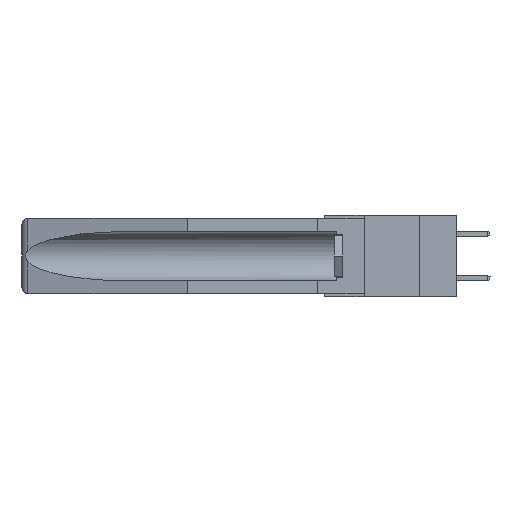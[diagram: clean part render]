
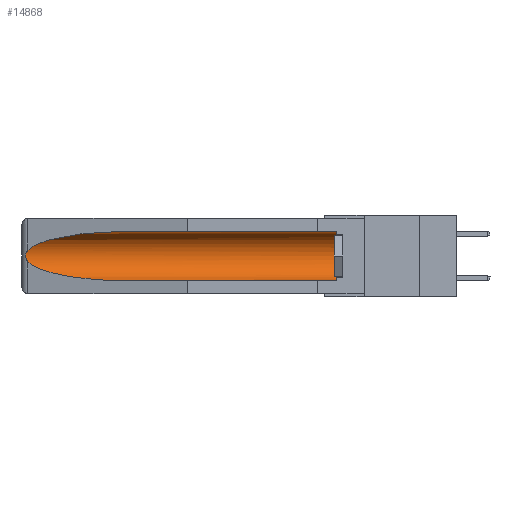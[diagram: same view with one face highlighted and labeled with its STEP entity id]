
A CAD part, left-side view. The second image highlights one B-rep face of the part: STEP entity #14868.
In plain terms, the highlighted cylindrical face has radius 2.857 mm (diameter 5.715 mm), a partial arc.
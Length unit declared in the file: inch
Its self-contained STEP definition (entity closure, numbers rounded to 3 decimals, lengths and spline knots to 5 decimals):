
#240 = CARTESIAN_POINT ( 'NONE',  ( 0.2675, 1.53308, -0.17534 ) ) ;
#1619 = ORIENTED_EDGE ( 'NONE', *, *, #8371, .F. ) ;
#1994 = VERTEX_POINT ( 'NONE', #13068 ) ;
#2024 = CARTESIAN_POINT ( 'NONE',  ( 0.26654, 1.53092, -0.15636 ) ) ;
#2436 = VERTEX_POINT ( 'NONE', #9187 ) ;
#3159 = LINE ( 'NONE', #11285, #17309 ) ;
#3239 =( BOUNDED_CURVE ( )  B_SPLINE_CURVE ( 3, ( #21529, #5232, #14236, #10741 ),
 .UNSPECIFIED., .F., .F. ) 
 B_SPLINE_CURVE_WITH_KNOTS ( ( 4, 4 ),
 ( 0.1948, 1.5708 ),
 .UNSPECIFIED. ) 
 CURVE ( )  GEOMETRIC_REPRESENTATION_ITEM ( )  RATIONAL_B_SPLINE_CURVE ( ( 1., 0.848, 0.848, 1. ) ) 
 REPRESENTATION_ITEM ( '' )  );
#3654 = CIRCLE ( 'NONE', #16038, 0.1125 ) ;
#4277 = EDGE_CURVE ( 'NONE', #15386, #20936, #3654, .T. ) ;
#4626 = ORIENTED_EDGE ( 'NONE', *, *, #18233, .T. ) ;
#5232 = CARTESIAN_POINT ( 'NONE',  ( 0.25451, 1.48313, -0.24835 ) ) ;
#5285 = CYLINDRICAL_SURFACE ( 'NONE', #21541, 0.1125 ) ;
#6024 = ORIENTED_EDGE ( 'NONE', *, *, #13712, .T. ) ;
#7390 = CARTESIAN_POINT ( 'NONE',  ( 0.26537, 1.52718, -0.19328 ) ) ;
#8225 = ORIENTED_EDGE ( 'NONE', *, *, #4277, .T. ) ;
#8371 = EDGE_CURVE ( 'NONE', #15386, #11142, #22810, .T. ) ;
#9187 = CARTESIAN_POINT ( 'NONE',  ( 0.26537, 1.52718, -0.14972 ) ) ;
#9372 = ORIENTED_EDGE ( 'NONE', *, *, #21915, .T. ) ;
#9944 = CARTESIAN_POINT ( 'NONE',  ( 0.155, 1.07973, -0.059 ) ) ;
#10266 = DIRECTION ( 'NONE',  ( 0., 0., 1. ) ) ;
#10741 = CARTESIAN_POINT ( 'NONE',  ( 0.155, 1.07973, -0.284 ) ) ;
#10810 = DIRECTION ( 'NONE',  ( 0., 1., 0. ) ) ;
#11142 = VERTEX_POINT ( 'NONE', #17273 ) ;
#11285 = CARTESIAN_POINT ( 'NONE',  ( 0.155, -0.30754, -0.059 ) ) ;
#11751 = CARTESIAN_POINT ( 'NONE',  ( 0.21114, 1.30732, -0.059 ) ) ;
#11768 = FACE_OUTER_BOUND ( 'NONE', #18163, .T. ) ;
#12874 = CARTESIAN_POINT ( 'NONE',  ( 0.2673, 1.53269, -0.17917 ) ) ;
#13068 = CARTESIAN_POINT ( 'NONE',  ( 0.155, 1.07973, -0.059 ) ) ;
#13133 = DIRECTION ( 'NONE',  ( 0., 1., 0. ) ) ;
#13134 = CARTESIAN_POINT ( 'NONE',  ( 0.26537, 1.52718, -0.19328 ) ) ;
#13282 = CARTESIAN_POINT ( 'NONE',  ( 0.26597, 1.5296, -0.19026 ) ) ;
#13712 = EDGE_CURVE ( 'NONE', #2436, #15270, #17717, .T. ) ;
#13774 = CARTESIAN_POINT ( 'NONE',  ( 0.155, 0.126, -0.1715 ) ) ;
#14236 = CARTESIAN_POINT ( 'NONE',  ( 0.21114, 1.30732, -0.284 ) ) ;
#14718 = CARTESIAN_POINT ( 'NONE',  ( 0.26655, 1.53094, -0.18657 ) ) ;
#14800 = CARTESIAN_POINT ( 'NONE',  ( 0.2675, 1.53308, -0.16763 ) ) ;
#14868 = ADVANCED_FACE ( 'NONE', ( #11768 ), #5285, .F. ) ;
#14964 = DIRECTION ( 'NONE',  ( 0., 0., 1. ) ) ;
#15035 = CARTESIAN_POINT ( 'NONE',  ( 0.155, -0.30754, -0.1715 ) ) ;
#15270 = VERTEX_POINT ( 'NONE', #7390 ) ;
#15386 = VERTEX_POINT ( 'NONE', #20463 ) ;
#16038 = AXIS2_PLACEMENT_3D ( 'NONE', #13774, #21041, #10266 ) ;
#16309 = CARTESIAN_POINT ( 'NONE',  ( 0.26597, 1.52961, -0.15275 ) ) ;
#16465 = CARTESIAN_POINT ( 'NONE',  ( 0.2673, 1.5327, -0.16383 ) ) ;
#16969 = CARTESIAN_POINT ( 'NONE',  ( 0.155, 0.126, -0.059 ) ) ;
#17189 = CARTESIAN_POINT ( 'NONE',  ( 0.26537, 1.52718, -0.14972 ) ) ;
#17273 = CARTESIAN_POINT ( 'NONE',  ( 0.155, 1.07973, -0.284 ) ) ;
#17309 = VECTOR ( 'NONE', #22815, 39.37008 ) ;
#17598 =( BOUNDED_CURVE ( )  B_SPLINE_CURVE ( 3, ( #9944, #11751, #19274, #17189 ),
 .UNSPECIFIED., .F., .F. ) 
 B_SPLINE_CURVE_WITH_KNOTS ( ( 4, 4 ),
 ( 4.71239, 6.08839 ),
 .UNSPECIFIED. ) 
 CURVE ( )  GEOMETRIC_REPRESENTATION_ITEM ( )  RATIONAL_B_SPLINE_CURVE ( ( 1., 0.848, 0.848, 1. ) ) 
 REPRESENTATION_ITEM ( '' )  );
#17644 = VECTOR ( 'NONE', #10810, 39.37008 ) ;
#17717 = B_SPLINE_CURVE_WITH_KNOTS ( 'NONE', 3,
 ( #21211, #16309, #2024, #16465, #14800, #240, #12874, #14718, #13282, #13134 ),
 .UNSPECIFIED., .F., .F.,
 ( 4, 2, 2, 2, 4 ),
 ( 0., 0.00029, 0.00058, 0.00087, 0.00117 ),
 .UNSPECIFIED. ) ;
#18163 = EDGE_LOOP ( 'NONE', ( #22425, #6024, #9372, #1619, #8225, #4626 ) ) ;
#18233 = EDGE_CURVE ( 'NONE', #20936, #1994, #3159, .T. ) ;
#19274 = CARTESIAN_POINT ( 'NONE',  ( 0.25451, 1.48313, -0.09465 ) ) ;
#19992 = CARTESIAN_POINT ( 'NONE',  ( 0.155, -0.30754, -0.284 ) ) ;
#20463 = CARTESIAN_POINT ( 'NONE',  ( 0.155, 0.126, -0.284 ) ) ;
#20936 = VERTEX_POINT ( 'NONE', #16969 ) ;
#21041 = DIRECTION ( 'NONE',  ( 0., -1., 0. ) ) ;
#21211 = CARTESIAN_POINT ( 'NONE',  ( 0.26537, 1.52718, -0.14972 ) ) ;
#21529 = CARTESIAN_POINT ( 'NONE',  ( 0.26537, 1.52718, -0.19328 ) ) ;
#21541 = AXIS2_PLACEMENT_3D ( 'NONE', #15035, #13133, #14964 ) ;
#21915 = EDGE_CURVE ( 'NONE', #15270, #11142, #3239, .T. ) ;
#22425 = ORIENTED_EDGE ( 'NONE', *, *, #22664, .T. ) ;
#22664 = EDGE_CURVE ( 'NONE', #1994, #2436, #17598, .T. ) ;
#22810 = LINE ( 'NONE', #19992, #17644 ) ;
#22815 = DIRECTION ( 'NONE',  ( 0., 1., 0. ) ) ;
